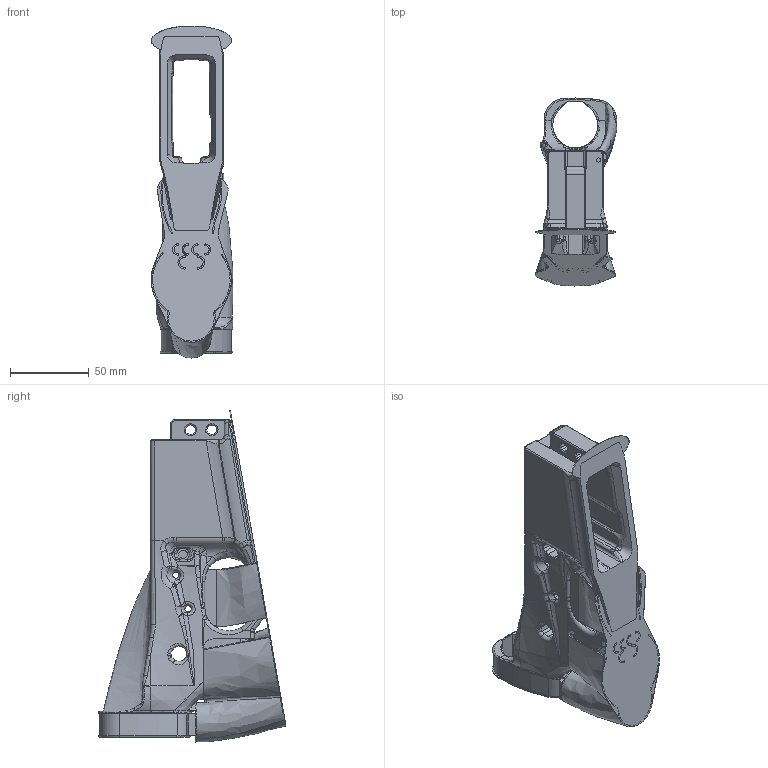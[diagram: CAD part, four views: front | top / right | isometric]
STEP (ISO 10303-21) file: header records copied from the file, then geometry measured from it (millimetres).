
FILE_DESCRIPTION (( 'STEP AP203' ), '1' );
FILE_NAME ('AR-15 BL V3.1 WS.STEP', '2022-05-05T17:12:57', ( '' ), ( '' ), 'SwSTEP 2.0', 'SolidWorks 2021', '' );
FILE_SCHEMA (( 'CONFIG_CONTROL_DESIGN' ));
Length unit declared in the file: inch
Products named in the file (1): AR-15 BL V3.1 WS
Bounding box: 51.89 x 119.27 x 210.65 mm (x, y, z)
Volume: 190369.6 mm3; surface area: 97938.4 mm2
Topology: 3 solids, 3 shells, 1997 faces, 5365 edges, 3394 vertices
Faces by surface type: bspline 773, plane 647, cylinder 436, torus 96, cone 30, sphere 15
Entity records: 127573 total; most frequent: CARTESIAN_POINT 84140, ORIENTED_EDGE 10650, DIRECTION 6705, EDGE_CURVE 5325, VERTEX_POINT 3394, AXIS2_PLACEMENT_3D 2259, VECTOR 2187, LINE 2187
